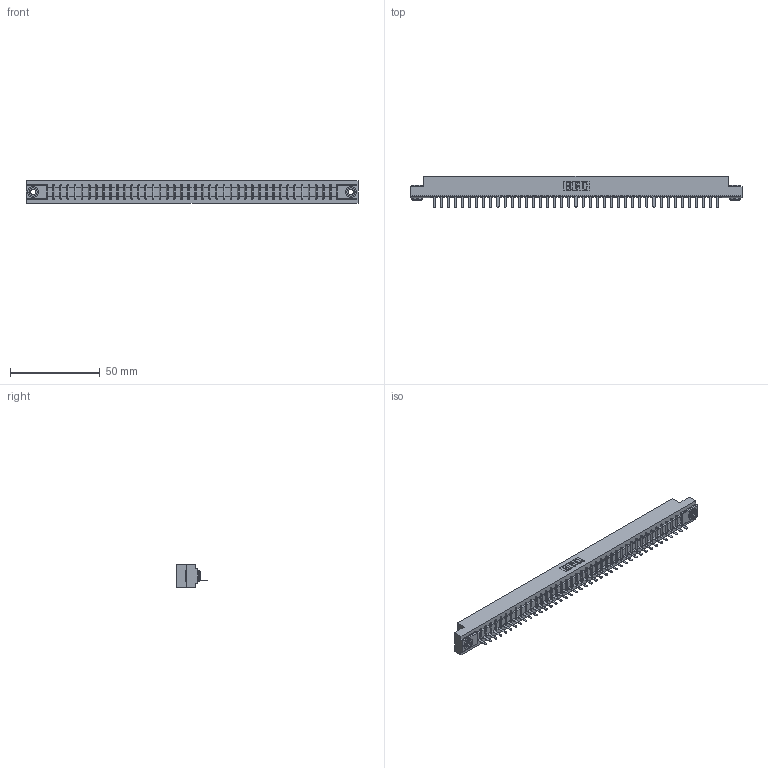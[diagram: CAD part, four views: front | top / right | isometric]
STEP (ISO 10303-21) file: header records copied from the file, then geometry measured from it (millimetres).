
FILE_DESCRIPTION (( 'STEP AP203' ), '1' );
FILE_NAME ('357-041-521-103.STEP', '2019-09-17T09:34:34', ( '' ), ( '' ), 'SwSTEP 2.0', 'SolidWorks 2016', '' );
FILE_SCHEMA (( 'CONFIG_CONTROL_DESIGN' ));
Length unit declared in the file: inch
Products named in the file (4): 307-290-002_521; 307 Part_.156 Dia Mounting Holes; 345-250-002_345-250-002-102; 357-041-521-103
Assembly tree (44 placements, depth 2):
  357-041-521-103
    307 Part_.156 Dia Mounting Holes
    307-290-002_521  x41
    345-250-002_345-250-002-102  x2
Bounding box: 185.47 x 17.42 x 12.7 mm (x, y, z)
Volume: 19844 mm3; surface area: 25185.1 mm2
Topology: 44 solids, 44 shells, 3246 faces, 9947 edges, 6514 vertices
Faces by surface type: plane 1939, cylinder 1215, sphere 84, cone 8
Entity records: 37055 total; most frequent: CARTESIAN_POINT 6229, ORIENTED_EDGE 6210, DIRECTION 6067, EDGE_CURVE 3105, LINE 2371, VECTOR 2371, VERTEX_POINT 2010, AXIS2_PLACEMENT_3D 1848
